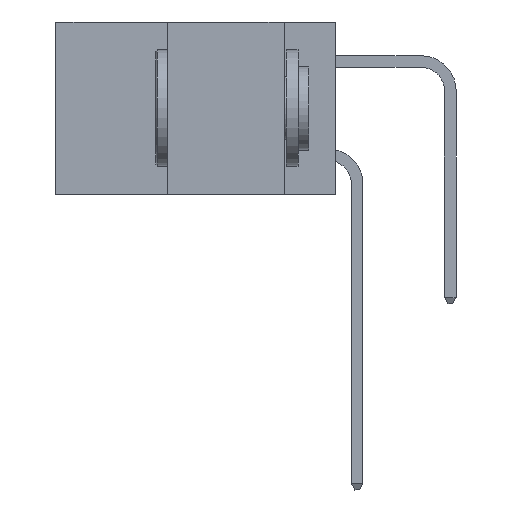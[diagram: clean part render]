
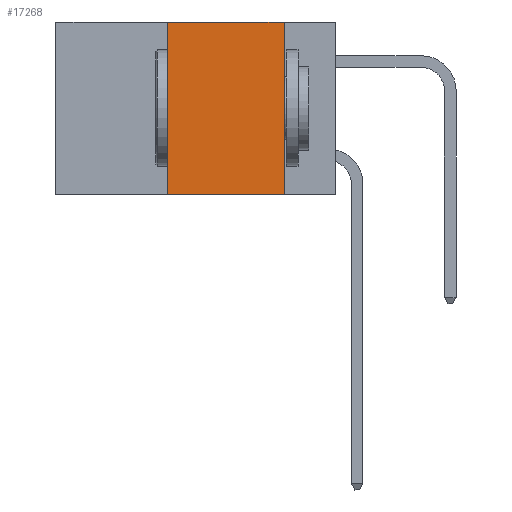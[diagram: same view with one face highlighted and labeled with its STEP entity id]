
A CAD part, left-side view. The second image highlights one B-rep face of the part: STEP entity #17268.
In plain terms, the highlighted planar face has unit normal (-1, 0, 0).
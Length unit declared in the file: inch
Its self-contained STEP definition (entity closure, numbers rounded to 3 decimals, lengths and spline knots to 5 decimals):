
#1704 = ORIENTED_EDGE ( 'NONE', *, *, #10685, .F. ) ;
#1720 = FACE_OUTER_BOUND ( 'NONE', #12420, .T. ) ;
#3459 = LINE ( 'NONE', #6968, #40328 ) ;
#3782 = EDGE_CURVE ( 'NONE', #40374, #18997, #39627, .T. ) ;
#4642 = DIRECTION ( 'NONE',  ( 1., 0., 0. ) ) ;
#5555 = ORIENTED_EDGE ( 'NONE', *, *, #3782, .F. ) ;
#5818 = DIRECTION ( 'NONE',  ( 0., 0., -1. ) ) ;
#6354 = DIRECTION ( 'NONE',  ( 0., -1., 0. ) ) ;
#6968 = CARTESIAN_POINT ( 'NONE',  ( 0., 0.6, 0. ) ) ;
#7007 = ORIENTED_EDGE ( 'NONE', *, *, #14843, .F. ) ;
#7572 = VERTEX_POINT ( 'NONE', #39041 ) ;
#8023 = LINE ( 'NONE', #14196, #11538 ) ;
#9055 = DIRECTION ( 'NONE',  ( 0., 0., 1. ) ) ;
#10299 = CARTESIAN_POINT ( 'NONE',  ( 0., 0.36, -0.37 ) ) ;
#10685 = EDGE_CURVE ( 'NONE', #7572, #35607, #8023, .T. ) ;
#11229 = VECTOR ( 'NONE', #9055, 39.37008 ) ;
#11538 = VECTOR ( 'NONE', #5818, 39.37008 ) ;
#12420 = EDGE_LOOP ( 'NONE', ( #1704, #7007, #5555, #16548 ) ) ;
#13464 = CARTESIAN_POINT ( 'NONE',  ( 0., 0.11, -0.37 ) ) ;
#13967 = PLANE ( 'NONE',  #24208 ) ;
#14196 = CARTESIAN_POINT ( 'NONE',  ( 0., 0.11, 0. ) ) ;
#14239 = CARTESIAN_POINT ( 'NONE',  ( 0., 0.6, 0. ) ) ;
#14355 = LINE ( 'NONE', #34598, #37763 ) ;
#14843 = EDGE_CURVE ( 'NONE', #18997, #7572, #3459, .T. ) ;
#16548 = ORIENTED_EDGE ( 'NONE', *, *, #21659, .T. ) ;
#17268 = ADVANCED_FACE ( 'NONE', ( #1720 ), #13967, .F. ) ;
#18997 = VERTEX_POINT ( 'NONE', #22304 ) ;
#21659 = EDGE_CURVE ( 'NONE', #40374, #35607, #14355, .T. ) ;
#22304 = CARTESIAN_POINT ( 'NONE',  ( 0., 0.36, 0. ) ) ;
#24208 = AXIS2_PLACEMENT_3D ( 'NONE', #14239, #4642, #29982 ) ;
#29527 = DIRECTION ( 'NONE',  ( 0., -1., 0. ) ) ;
#29982 = DIRECTION ( 'NONE',  ( 0., 0., -1. ) ) ;
#31081 = CARTESIAN_POINT ( 'NONE',  ( 0., 0.36, 0. ) ) ;
#34598 = CARTESIAN_POINT ( 'NONE',  ( 0., 0.6, -0.37 ) ) ;
#35607 = VERTEX_POINT ( 'NONE', #13464 ) ;
#37763 = VECTOR ( 'NONE', #6354, 39.37008 ) ;
#39041 = CARTESIAN_POINT ( 'NONE',  ( 0., 0.11, 0. ) ) ;
#39627 = LINE ( 'NONE', #31081, #11229 ) ;
#40328 = VECTOR ( 'NONE', #29527, 39.37008 ) ;
#40374 = VERTEX_POINT ( 'NONE', #10299 ) ;
